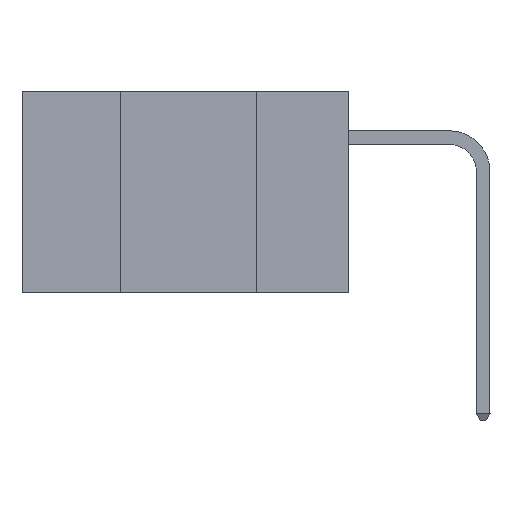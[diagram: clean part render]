
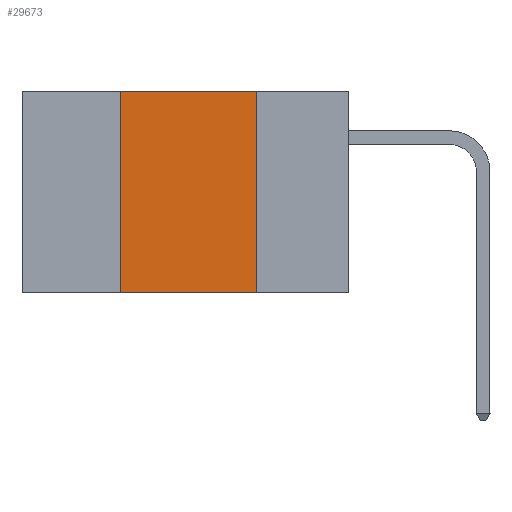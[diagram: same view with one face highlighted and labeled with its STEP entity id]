
A CAD part, left-side view. The second image highlights one B-rep face of the part: STEP entity #29673.
In plain terms, the highlighted planar face has unit normal (-1, 0, 0).
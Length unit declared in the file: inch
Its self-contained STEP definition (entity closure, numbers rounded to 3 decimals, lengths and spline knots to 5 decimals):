
#877 = VECTOR ( 'NONE', #10282, 39.37008 ) ;
#878 = DIRECTION ( 'NONE',  ( 0., 0., -1. ) ) ;
#1768 = VECTOR ( 'NONE', #27651, 39.37008 ) ;
#2069 = CARTESIAN_POINT ( 'NONE',  ( 0., 0.6, -0.37 ) ) ;
#4394 = ORIENTED_EDGE ( 'NONE', *, *, #27550, .T. ) ;
#5539 = DIRECTION ( 'NONE',  ( 0., 0., -1. ) ) ;
#5913 = VERTEX_POINT ( 'NONE', #7154 ) ;
#6457 = ORIENTED_EDGE ( 'NONE', *, *, #9241, .F. ) ;
#7154 = CARTESIAN_POINT ( 'NONE',  ( 0., 0.17, 0. ) ) ;
#7866 = VECTOR ( 'NONE', #878, 39.37008 ) ;
#8392 = AXIS2_PLACEMENT_3D ( 'NONE', #19234, #21457, #5539 ) ;
#9241 = EDGE_CURVE ( 'NONE', #18980, #5913, #17338, .T. ) ;
#10282 = DIRECTION ( 'NONE',  ( 0., 0., 1. ) ) ;
#11389 = CARTESIAN_POINT ( 'NONE',  ( 0., 0.17, 0. ) ) ;
#12048 = EDGE_CURVE ( 'NONE', #17412, #18980, #17897, .T. ) ;
#13668 = FACE_OUTER_BOUND ( 'NONE', #17860, .T. ) ;
#16533 = PLANE ( 'NONE',  #8392 ) ;
#17173 = CARTESIAN_POINT ( 'NONE',  ( 0., 0.6, 0. ) ) ;
#17338 = LINE ( 'NONE', #17173, #33303 ) ;
#17412 = VERTEX_POINT ( 'NONE', #28486 ) ;
#17860 = EDGE_LOOP ( 'NONE', ( #30245, #6457, #25416, #4394 ) ) ;
#17897 = LINE ( 'NONE', #33473, #877 ) ;
#18980 = VERTEX_POINT ( 'NONE', #30988 ) ;
#19234 = CARTESIAN_POINT ( 'NONE',  ( 0., 0.6, 0. ) ) ;
#20384 = DIRECTION ( 'NONE',  ( 0., -1., 0. ) ) ;
#21457 = DIRECTION ( 'NONE',  ( 1., 0., 0. ) ) ;
#21986 = VERTEX_POINT ( 'NONE', #22370 ) ;
#22370 = CARTESIAN_POINT ( 'NONE',  ( 0., 0.17, -0.37 ) ) ;
#25416 = ORIENTED_EDGE ( 'NONE', *, *, #12048, .F. ) ;
#26792 = LINE ( 'NONE', #11389, #7866 ) ;
#27550 = EDGE_CURVE ( 'NONE', #17412, #21986, #30509, .T. ) ;
#27651 = DIRECTION ( 'NONE',  ( 0., -1., 0. ) ) ;
#28486 = CARTESIAN_POINT ( 'NONE',  ( 0., 0.42, -0.37 ) ) ;
#29673 = ADVANCED_FACE ( 'NONE', ( #13668 ), #16533, .F. ) ;
#30245 = ORIENTED_EDGE ( 'NONE', *, *, #31656, .F. ) ;
#30509 = LINE ( 'NONE', #2069, #1768 ) ;
#30988 = CARTESIAN_POINT ( 'NONE',  ( 0., 0.42, 0. ) ) ;
#31656 = EDGE_CURVE ( 'NONE', #5913, #21986, #26792, .T. ) ;
#33303 = VECTOR ( 'NONE', #20384, 39.37008 ) ;
#33473 = CARTESIAN_POINT ( 'NONE',  ( 0., 0.42, 0. ) ) ;
